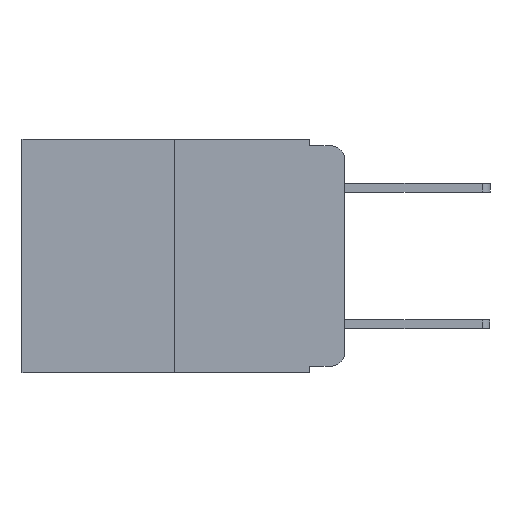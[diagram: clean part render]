
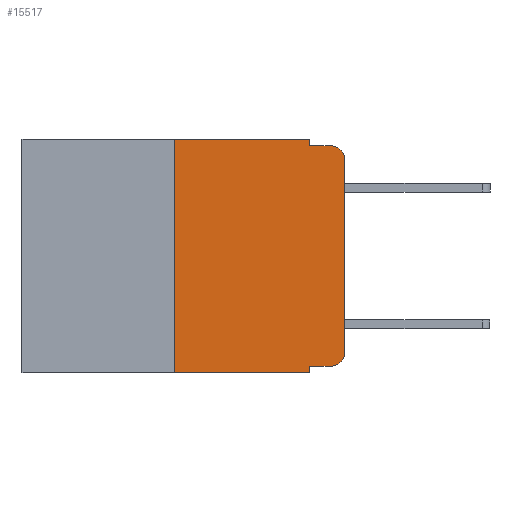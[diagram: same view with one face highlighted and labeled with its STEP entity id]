
A CAD part, left-side view. The second image highlights one B-rep face of the part: STEP entity #15517.
In plain terms, the highlighted planar face has unit normal (-1, 0, 0).
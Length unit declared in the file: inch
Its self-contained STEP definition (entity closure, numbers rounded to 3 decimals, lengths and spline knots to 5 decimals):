
#540 = CARTESIAN_POINT ( 'NONE',  ( 0., 0.051, -0.343 ) ) ;
#578 = DIRECTION ( 'NONE',  ( 0., 0., 1. ) ) ;
#1102 = VECTOR ( 'NONE', #8694, 39.37008 ) ;
#1239 = AXIS2_PLACEMENT_3D ( 'NONE', #14518, #6366, #15906 ) ;
#1926 = CARTESIAN_POINT ( 'NONE',  ( 0., 0., 0. ) ) ;
#1934 = VECTOR ( 'NONE', #4489, 39.37008 ) ;
#2137 = CARTESIAN_POINT ( 'NONE',  ( 0., 0., -0.03 ) ) ;
#3352 = VECTOR ( 'NONE', #578, 39.37008 ) ;
#3999 = DIRECTION ( 'NONE',  ( -1., 0., 0. ) ) ;
#4032 = AXIS2_PLACEMENT_3D ( 'NONE', #12179, #3999, #13562 ) ;
#4289 = EDGE_CURVE ( 'NONE', #9779, #14302, #8855, .T. ) ;
#4489 = DIRECTION ( 'NONE',  ( 0., -1., 0. ) ) ;
#4622 = ORIENTED_EDGE ( 'NONE', *, *, #9680, .F. ) ;
#4638 = DIRECTION ( 'NONE',  ( 1., 0., 0. ) ) ;
#4745 = CARTESIAN_POINT ( 'NONE',  ( 0., 0.473, 0. ) ) ;
#4857 = ORIENTED_EDGE ( 'NONE', *, *, #4289, .F. ) ;
#5748 = VECTOR ( 'NONE', #12926, 39.37008 ) ;
#5909 = ORIENTED_EDGE ( 'NONE', *, *, #16866, .F. ) ;
#5959 = LINE ( 'NONE', #9847, #9163 ) ;
#6366 = DIRECTION ( 'NONE',  ( -1., 0., 0. ) ) ;
#6419 = FACE_OUTER_BOUND ( 'NONE', #10033, .T. ) ;
#6467 = VERTEX_POINT ( 'NONE', #16116 ) ;
#6524 = CARTESIAN_POINT ( 'NONE',  ( 0., 0.25, 0. ) ) ;
#6536 = ORIENTED_EDGE ( 'NONE', *, *, #16407, .F. ) ;
#7027 = LINE ( 'NONE', #1926, #3352 ) ;
#7184 = DIRECTION ( 'NONE',  ( 0., -1., 0. ) ) ;
#7470 = EDGE_CURVE ( 'NONE', #9660, #11554, #13499, .T. ) ;
#7623 = ORIENTED_EDGE ( 'NONE', *, *, #14194, .T. ) ;
#8019 = VERTEX_POINT ( 'NONE', #2137 ) ;
#8035 = ORIENTED_EDGE ( 'NONE', *, *, #9815, .T. ) ;
#8124 = DIRECTION ( 'NONE',  ( 0., -1., 0. ) ) ;
#8213 = VERTEX_POINT ( 'NONE', #13496 ) ;
#8219 = VECTOR ( 'NONE', #8124, 39.37008 ) ;
#8369 = VERTEX_POINT ( 'NONE', #11170 ) ;
#8694 = DIRECTION ( 'NONE',  ( 0., 0., -1. ) ) ;
#8718 = VECTOR ( 'NONE', #9549, 39.37008 ) ;
#8855 = LINE ( 'NONE', #17478, #1102 ) ;
#8943 = LINE ( 'NONE', #4745, #5748 ) ;
#9163 = VECTOR ( 'NONE', #7184, 39.37008 ) ;
#9444 = VECTOR ( 'NONE', #17408, 39.37008 ) ;
#9549 = DIRECTION ( 'NONE',  ( 0., 0., 1. ) ) ;
#9660 = VERTEX_POINT ( 'NONE', #10108 ) ;
#9680 = EDGE_CURVE ( 'NONE', #16160, #9660, #8943, .T. ) ;
#9761 = ORIENTED_EDGE ( 'NONE', *, *, #12788, .T. ) ;
#9779 = VERTEX_POINT ( 'NONE', #14416 ) ;
#9815 = EDGE_CURVE ( 'NONE', #8019, #6467, #14491, .T. ) ;
#9847 = CARTESIAN_POINT ( 'NONE',  ( 0., 0.051, -0.01 ) ) ;
#9946 = ORIENTED_EDGE ( 'NONE', *, *, #16542, .T. ) ;
#10033 = EDGE_LOOP ( 'NONE', ( #9946, #8035, #6536, #10605, #4622, #5909, #7623, #4857, #9761, #10622 ) ) ;
#10052 = PLANE ( 'NONE',  #11269 ) ;
#10108 = CARTESIAN_POINT ( 'NONE',  ( 0., 0.051, 0. ) ) ;
#10605 = ORIENTED_EDGE ( 'NONE', *, *, #7470, .F. ) ;
#10622 = ORIENTED_EDGE ( 'NONE', *, *, #14583, .T. ) ;
#11170 = CARTESIAN_POINT ( 'NONE',  ( 0., 0.25, -0.343 ) ) ;
#11249 = CARTESIAN_POINT ( 'NONE',  ( 0., 0.473, -0.343 ) ) ;
#11269 = AXIS2_PLACEMENT_3D ( 'NONE', #12810, #4638, #14183 ) ;
#11402 = LINE ( 'NONE', #16302, #8219 ) ;
#11554 = VERTEX_POINT ( 'NONE', #11675 ) ;
#11675 = CARTESIAN_POINT ( 'NONE',  ( 0., 0.051, -0.01 ) ) ;
#12179 = CARTESIAN_POINT ( 'NONE',  ( 0., 0.02, -0.313 ) ) ;
#12349 = LINE ( 'NONE', #17704, #8718 ) ;
#12788 = EDGE_CURVE ( 'NONE', #9779, #8213, #11402, .T. ) ;
#12810 = CARTESIAN_POINT ( 'NONE',  ( 0., 0.473, 0. ) ) ;
#12926 = DIRECTION ( 'NONE',  ( 0., -1., 0. ) ) ;
#13277 = CIRCLE ( 'NONE', #4032, 0.02 ) ;
#13496 = CARTESIAN_POINT ( 'NONE',  ( 0., 0.02, -0.333 ) ) ;
#13499 = LINE ( 'NONE', #16035, #9444 ) ;
#13562 = DIRECTION ( 'NONE',  ( 0., 0., -1. ) ) ;
#14183 = DIRECTION ( 'NONE',  ( 0., 0., -1. ) ) ;
#14194 = EDGE_CURVE ( 'NONE', #8369, #14302, #16508, .T. ) ;
#14302 = VERTEX_POINT ( 'NONE', #540 ) ;
#14416 = CARTESIAN_POINT ( 'NONE',  ( 0., 0.051, -0.333 ) ) ;
#14491 = CIRCLE ( 'NONE', #1239, 0.02 ) ;
#14518 = CARTESIAN_POINT ( 'NONE',  ( 0., 0.02, -0.03 ) ) ;
#14583 = EDGE_CURVE ( 'NONE', #8213, #16707, #13277, .T. ) ;
#15517 = ADVANCED_FACE ( 'NONE', ( #6419 ), #10052, .F. ) ;
#15906 = DIRECTION ( 'NONE',  ( 0., 0., -1. ) ) ;
#16035 = CARTESIAN_POINT ( 'NONE',  ( 0., 0.051, 0. ) ) ;
#16116 = CARTESIAN_POINT ( 'NONE',  ( 0., 0.02, -0.01 ) ) ;
#16160 = VERTEX_POINT ( 'NONE', #6524 ) ;
#16302 = CARTESIAN_POINT ( 'NONE',  ( 0., 0.051, -0.333 ) ) ;
#16407 = EDGE_CURVE ( 'NONE', #11554, #6467, #5959, .T. ) ;
#16508 = LINE ( 'NONE', #11249, #1934 ) ;
#16542 = EDGE_CURVE ( 'NONE', #16707, #8019, #7027, .T. ) ;
#16707 = VERTEX_POINT ( 'NONE', #17358 ) ;
#16866 = EDGE_CURVE ( 'NONE', #8369, #16160, #12349, .T. ) ;
#17358 = CARTESIAN_POINT ( 'NONE',  ( 0., 0., -0.313 ) ) ;
#17408 = DIRECTION ( 'NONE',  ( 0., 0., -1. ) ) ;
#17478 = CARTESIAN_POINT ( 'NONE',  ( 0., 0.051, 0. ) ) ;
#17704 = CARTESIAN_POINT ( 'NONE',  ( 0., 0.25, 0. ) ) ;
